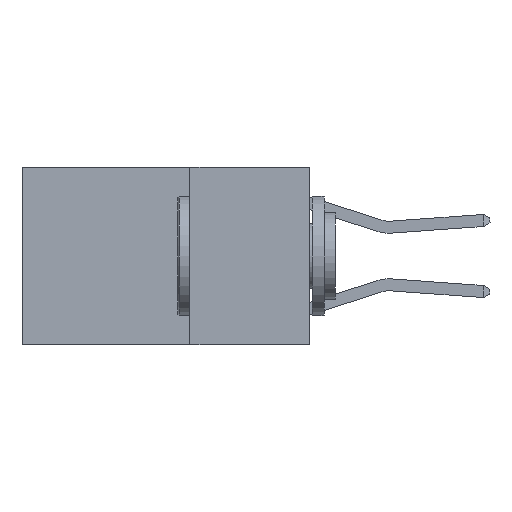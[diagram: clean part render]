
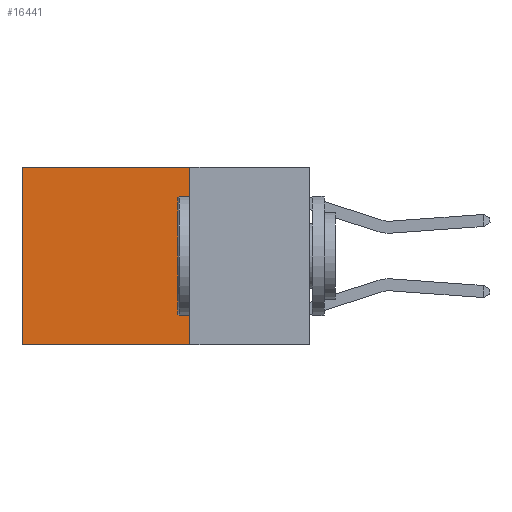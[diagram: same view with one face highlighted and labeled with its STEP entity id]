
A CAD part, left-side view. The second image highlights one B-rep face of the part: STEP entity #16441.
In plain terms, the highlighted planar face has unit normal (-1, 0, 0).
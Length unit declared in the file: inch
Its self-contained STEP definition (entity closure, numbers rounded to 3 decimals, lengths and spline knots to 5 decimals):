
#216 = ORIENTED_EDGE ( 'NONE', *, *, #17860, .T. ) ;
#687 = CARTESIAN_POINT ( 'NONE',  ( 0.2625, 0.25, 0. ) ) ;
#974 = CARTESIAN_POINT ( 'NONE',  ( 0.2625, 0.6, 0. ) ) ;
#1047 = EDGE_CURVE ( 'NONE', #10232, #17008, #14069, .T. ) ;
#1735 = FACE_OUTER_BOUND ( 'NONE', #5087, .T. ) ;
#2185 = DIRECTION ( 'NONE',  ( 0., 1., 0. ) ) ;
#2273 = DIRECTION ( 'NONE',  ( 0., 0., -1. ) ) ;
#2607 = CARTESIAN_POINT ( 'NONE',  ( 0.2625, 0.25, -0.37 ) ) ;
#2946 = EDGE_CURVE ( 'NONE', #8613, #8929, #4069, .T. ) ;
#3226 = EDGE_CURVE ( 'NONE', #10232, #8613, #15914, .T. ) ;
#3755 = CARTESIAN_POINT ( 'NONE',  ( 0.2625, 0.25, 0. ) ) ;
#3826 = VECTOR ( 'NONE', #10584, 39.37008 ) ;
#4069 = LINE ( 'NONE', #16179, #20351 ) ;
#5087 = EDGE_LOOP ( 'NONE', ( #216, #11444, #19280, #12950 ) ) ;
#8598 = CARTESIAN_POINT ( 'NONE',  ( 0.2625, 0.6, 0. ) ) ;
#8601 = CARTESIAN_POINT ( 'NONE',  ( 0.2625, 0.25, 0. ) ) ;
#8613 = VERTEX_POINT ( 'NONE', #2607 ) ;
#8929 = VERTEX_POINT ( 'NONE', #12873 ) ;
#8991 = CARTESIAN_POINT ( 'NONE',  ( 0.2625, 0.25, 0. ) ) ;
#9855 = VECTOR ( 'NONE', #2185, 39.37008 ) ;
#9861 = LINE ( 'NONE', #974, #17232 ) ;
#10232 = VERTEX_POINT ( 'NONE', #8601 ) ;
#10361 = DIRECTION ( 'NONE',  ( 0., 0., -1. ) ) ;
#10584 = DIRECTION ( 'NONE',  ( 0., 0., -1. ) ) ;
#11444 = ORIENTED_EDGE ( 'NONE', *, *, #2946, .F. ) ;
#11765 = DIRECTION ( 'NONE',  ( 1., 0., 0. ) ) ;
#12873 = CARTESIAN_POINT ( 'NONE',  ( 0.2625, 0.6, -0.37 ) ) ;
#12950 = ORIENTED_EDGE ( 'NONE', *, *, #1047, .T. ) ;
#14069 = LINE ( 'NONE', #3755, #9855 ) ;
#15914 = LINE ( 'NONE', #8991, #3826 ) ;
#16179 = CARTESIAN_POINT ( 'NONE',  ( 0.2625, 0.25, -0.37 ) ) ;
#16441 = ADVANCED_FACE ( 'NONE', ( #1735 ), #17992, .F. ) ;
#16512 = AXIS2_PLACEMENT_3D ( 'NONE', #687, #11765, #2273 ) ;
#17008 = VERTEX_POINT ( 'NONE', #8598 ) ;
#17232 = VECTOR ( 'NONE', #10361, 39.37008 ) ;
#17831 = DIRECTION ( 'NONE',  ( 0., 1., 0. ) ) ;
#17860 = EDGE_CURVE ( 'NONE', #17008, #8929, #9861, .T. ) ;
#17992 = PLANE ( 'NONE',  #16512 ) ;
#19280 = ORIENTED_EDGE ( 'NONE', *, *, #3226, .F. ) ;
#20351 = VECTOR ( 'NONE', #17831, 39.37008 ) ;
